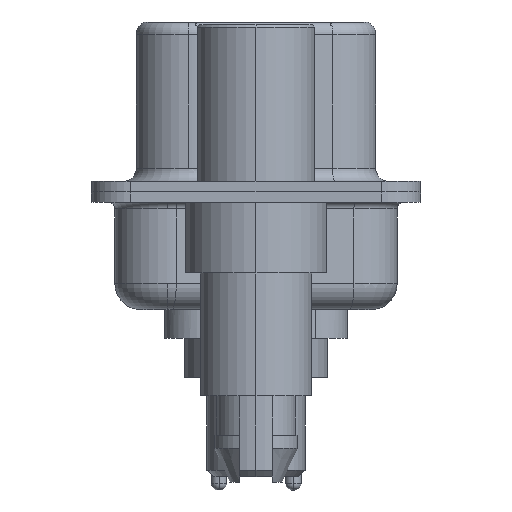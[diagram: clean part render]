
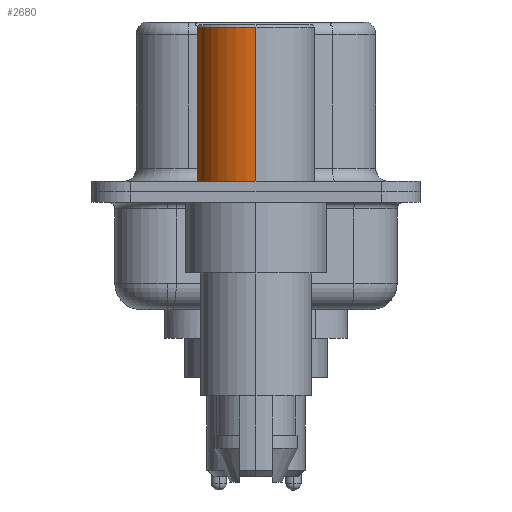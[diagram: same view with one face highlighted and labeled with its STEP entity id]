
A CAD part, left-side view. The second image highlights one B-rep face of the part: STEP entity #2680.
In plain terms, the highlighted cylindrical face has radius 2.25 mm (diameter 4.5 mm), a partial arc.
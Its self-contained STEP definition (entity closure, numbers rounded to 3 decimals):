
#766 = AXIS2_PLACEMENT_3D ( 'NONE', #17061, #4785, #19146 ) ;
#1565 = CARTESIAN_POINT ( 'NONE',  ( -2.25, 0., 0.581 ) ) ;
#2317 = CIRCLE ( 'NONE', #5699, 2.25 ) ;
#2680 = ADVANCED_FACE ( 'NONE', ( #19539 ), #3130, .T. ) ;
#3029 = ORIENTED_EDGE ( 'NONE', *, *, #21404, .F. ) ;
#3130 = CYLINDRICAL_SURFACE ( 'NONE', #11978, 2.25 ) ;
#3271 = DIRECTION ( 'NONE',  ( 0., 0., 1. ) ) ;
#4785 = DIRECTION ( 'NONE',  ( 0., 0., 1. ) ) ;
#5603 = ORIENTED_EDGE ( 'NONE', *, *, #26118, .F. ) ;
#5606 = LINE ( 'NONE', #18949, #15862 ) ;
#5699 = AXIS2_PLACEMENT_3D ( 'NONE', #15578, #3271, #17647 ) ;
#5872 = EDGE_LOOP ( 'NONE', ( #6089, #23223, #5603, #3029 ) ) ;
#6089 = ORIENTED_EDGE ( 'NONE', *, *, #18601, .T. ) ;
#6582 = VERTEX_POINT ( 'NONE', #9191 ) ;
#7066 = CARTESIAN_POINT ( 'NONE',  ( -2.25, 0., 6.3 ) ) ;
#8452 = CARTESIAN_POINT ( 'NONE',  ( -2.25, 0., 0.4 ) ) ;
#9191 = CARTESIAN_POINT ( 'NONE',  ( 2.25, 0., 6.3 ) ) ;
#11978 = AXIS2_PLACEMENT_3D ( 'NONE', #26585, #21384, #22703 ) ;
#12164 = VERTEX_POINT ( 'NONE', #24566 ) ;
#12258 = VERTEX_POINT ( 'NONE', #8452 ) ;
#15578 = CARTESIAN_POINT ( 'NONE',  ( 0., 0., 6.3 ) ) ;
#15862 = VECTOR ( 'NONE', #21041, 1000. ) ;
#15971 = DIRECTION ( 'NONE',  ( 0., 0., 1. ) ) ;
#17061 = CARTESIAN_POINT ( 'NONE',  ( 0., 0., 0.4 ) ) ;
#17118 = VERTEX_POINT ( 'NONE', #7066 ) ;
#17472 = LINE ( 'NONE', #1565, #18115 ) ;
#17647 = DIRECTION ( 'NONE',  ( 1., 0., 0. ) ) ;
#18115 = VECTOR ( 'NONE', #15971, 1000. ) ;
#18601 = EDGE_CURVE ( 'NONE', #12164, #12258, #22782, .T. ) ;
#18949 = CARTESIAN_POINT ( 'NONE',  ( 2.25, 0., 0.581 ) ) ;
#19146 = DIRECTION ( 'NONE',  ( 1., 0., 0. ) ) ;
#19539 = FACE_OUTER_BOUND ( 'NONE', #5872, .T. ) ;
#21041 = DIRECTION ( 'NONE',  ( 0., 0., 1. ) ) ;
#21384 = DIRECTION ( 'NONE',  ( 0., 0., 1. ) ) ;
#21404 = EDGE_CURVE ( 'NONE', #12164, #6582, #5606, .T. ) ;
#22703 = DIRECTION ( 'NONE',  ( 1., 0., 0. ) ) ;
#22782 = CIRCLE ( 'NONE', #766, 2.25 ) ;
#23223 = ORIENTED_EDGE ( 'NONE', *, *, #25612, .T. ) ;
#24566 = CARTESIAN_POINT ( 'NONE',  ( 2.25, 0., 0.4 ) ) ;
#25612 = EDGE_CURVE ( 'NONE', #12258, #17118, #17472, .T. ) ;
#26118 = EDGE_CURVE ( 'NONE', #6582, #17118, #2317, .T. ) ;
#26585 = CARTESIAN_POINT ( 'NONE',  ( 0., 0., 0.581 ) ) ;
